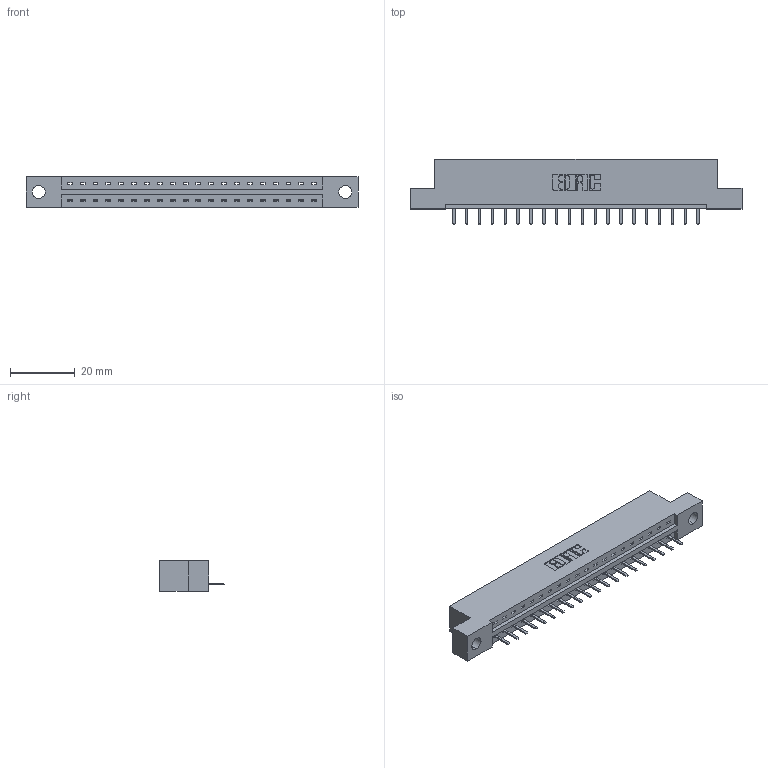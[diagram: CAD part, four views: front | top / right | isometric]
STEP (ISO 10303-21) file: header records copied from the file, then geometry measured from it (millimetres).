
FILE_DESCRIPTION (( 'STEP AP203' ), '1' );
FILE_NAME ('387-020-520-104.STEP', '2019-10-02T22:02:18', ( '' ), ( '' ), 'SwSTEP 2.0', 'SolidWorks 2016', '' );
FILE_SCHEMA (( 'CONFIG_CONTROL_DESIGN' ));
Length unit declared in the file: inch
Products named in the file (3): 387-020-520-104; 345-292-001_345-293-120; 337 Part_Flush Mounting Lugs - 0.156 Dia-TH
Assembly tree (21 placements, depth 2):
  387-020-520-104
    337 Part_Flush Mounting Lugs - 0.156 Dia-TH
    345-292-001_345-293-120  x20
Bounding box: 102.26 x 20.02 x 9.4 mm (x, y, z)
Volume: 10207.6 mm3; surface area: 10014.1 mm2
Topology: 21 solids, 21 shells, 1434 faces, 4231 edges, 2766 vertices
Faces by surface type: plane 1030, cylinder 404
Entity records: 17829 total; most frequent: CARTESIAN_POINT 3122, ORIENTED_EDGE 3066, DIRECTION 2661, EDGE_CURVE 1533, VECTOR 1401, LINE 1401, VERTEX_POINT 1018, AXIS2_PLACEMENT_3D 630
